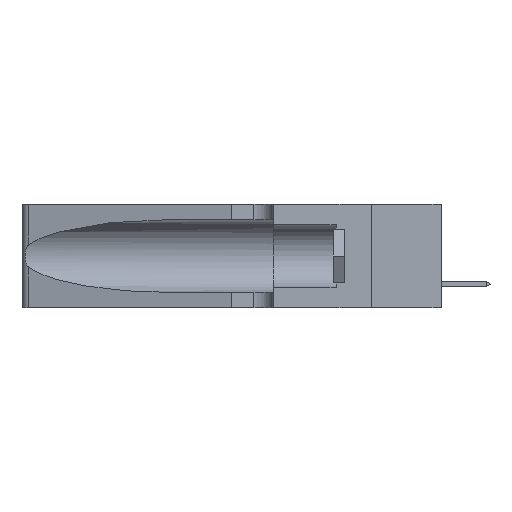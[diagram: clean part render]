
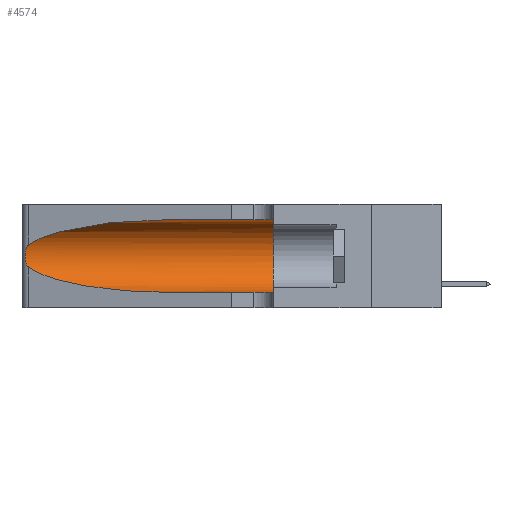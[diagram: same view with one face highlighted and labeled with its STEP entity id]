
A CAD part, left-side view. The second image highlights one B-rep face of the part: STEP entity #4574.
In plain terms, the highlighted cylindrical face has radius 3.308 mm (diameter 6.617 mm), a partial arc.
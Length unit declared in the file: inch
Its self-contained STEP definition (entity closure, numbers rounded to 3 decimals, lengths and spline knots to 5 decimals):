
#423 = CARTESIAN_POINT ( 'NONE',  ( 0.1305, 1.61858, 0.05475 ) ) ;
#582 = FACE_OUTER_BOUND ( 'NONE', #7957, .T. ) ;
#1213 = VERTEX_POINT ( 'NONE', #10068 ) ;
#1557 = EDGE_CURVE ( 'NONE', #7163, #1213, #6737, .T. ) ;
#1610 = CARTESIAN_POINT ( 'NONE',  ( 0.1305, 0.72297, 0.31525 ) ) ;
#2842 = CARTESIAN_POINT ( 'NONE',  ( 0.2373, 1.15595, 0.28018 ) ) ;
#3681 = ORIENTED_EDGE ( 'NONE', *, *, #4678, .T. ) ;
#3948 = CARTESIAN_POINT ( 'NONE',  ( 0.25787, 1.23484, 0.2124 ) ) ;
#4024 = CARTESIAN_POINT ( 'NONE',  ( 0.25555, 1.22993, 0.14849 ) ) ;
#4443 = ORIENTED_EDGE ( 'NONE', *, *, #22058, .F. ) ;
#4574 = ADVANCED_FACE ( 'NONE', ( #582 ), #6459, .F. ) ;
#4678 = EDGE_CURVE ( 'NONE', #1213, #16218, #20661, .T. ) ;
#4921 = CARTESIAN_POINT ( 'NONE',  ( 0.25487, 1.22718, 0.14631 ) ) ;
#6112 = CARTESIAN_POINT ( 'NONE',  ( 0.25487, 1.22718, 0.22369 ) ) ;
#6451 = VECTOR ( 'NONE', #15486, 39.37008 ) ;
#6459 = CYLINDRICAL_SURFACE ( 'NONE', #15802, 0.13025 ) ;
#6737 =( BOUNDED_CURVE ( )  B_SPLINE_CURVE ( 3, ( #4921, #11575, #7399, #14193 ),
 .UNSPECIFIED., .F., .T. ) 
 B_SPLINE_CURVE_WITH_KNOTS ( ( 4, 4 ),
 ( 3.44316, 4.71239 ),
 .UNSPECIFIED. ) 
 CURVE ( )  GEOMETRIC_REPRESENTATION_ITEM ( )  RATIONAL_B_SPLINE_CURVE ( ( 1., 0.87, 0.87, 1. ) ) 
 REPRESENTATION_ITEM ( '' )  );
#7163 = VERTEX_POINT ( 'NONE', #8894 ) ;
#7164 = CARTESIAN_POINT ( 'NONE',  ( 0.25487, 1.22718, 0.22369 ) ) ;
#7399 = CARTESIAN_POINT ( 'NONE',  ( 0.18966, 0.96281, 0.05475 ) ) ;
#7523 = DIRECTION ( 'NONE',  ( 0., 0., -1. ) ) ;
#7957 = EDGE_LOOP ( 'NONE', ( #8429, #14013, #21726, #3681, #17654, #4443 ) ) ;
#8325 = LINE ( 'NONE', #15269, #6451 ) ;
#8429 = ORIENTED_EDGE ( 'NONE', *, *, #15650, .T. ) ;
#8894 = CARTESIAN_POINT ( 'NONE',  ( 0.25487, 1.22718, 0.14631 ) ) ;
#9244 = VERTEX_POINT ( 'NONE', #6112 ) ;
#10068 = CARTESIAN_POINT ( 'NONE',  ( 0.1305, 0.72297, 0.05475 ) ) ;
#10772 = CARTESIAN_POINT ( 'NONE',  ( 0.25856, 1.23593, 0.16098 ) ) ;
#11281 = CARTESIAN_POINT ( 'NONE',  ( 0.25487, 1.22718, 0.22369 ) ) ;
#11575 = CARTESIAN_POINT ( 'NONE',  ( 0.2373, 1.15595, 0.08982 ) ) ;
#12140 = EDGE_CURVE ( 'NONE', #9244, #7163, #19660, .T. ) ;
#12554 = CARTESIAN_POINT ( 'NONE',  ( 0.26075, 1.23896, 0.178 ) ) ;
#12938 = AXIS2_PLACEMENT_3D ( 'NONE', #17990, #21541, #21406 ) ;
#13100 = CARTESIAN_POINT ( 'NONE',  ( 0.18966, 0.96281, 0.31525 ) ) ;
#13196 = VERTEX_POINT ( 'NONE', #1610 ) ;
#14013 = ORIENTED_EDGE ( 'NONE', *, *, #12140, .T. ) ;
#14113 = CARTESIAN_POINT ( 'NONE',  ( 0.25555, 1.22994, 0.2215 ) ) ;
#14164 = DIRECTION ( 'NONE',  ( 0., -1., 0. ) ) ;
#14193 = CARTESIAN_POINT ( 'NONE',  ( 0.1305, 0.72297, 0.05475 ) ) ;
#14201 = CARTESIAN_POINT ( 'NONE',  ( 0.25639, 1.23184, 0.21858 ) ) ;
#14276 = CARTESIAN_POINT ( 'NONE',  ( 0.25639, 1.23186, 0.15144 ) ) ;
#14664 = VERTEX_POINT ( 'NONE', #15324 ) ;
#14884 = CIRCLE ( 'NONE', #12938, 0.13025 ) ;
#15269 = CARTESIAN_POINT ( 'NONE',  ( 0.1305, 1.61858, 0.31525 ) ) ;
#15324 = CARTESIAN_POINT ( 'NONE',  ( 0.1305, 0.35, 0.31525 ) ) ;
#15486 = DIRECTION ( 'NONE',  ( 0., -1., 0. ) ) ;
#15650 = EDGE_CURVE ( 'NONE', #13196, #9244, #18834, .T. ) ;
#15802 = AXIS2_PLACEMENT_3D ( 'NONE', #19537, #14164, #7523 ) ;
#15947 = CARTESIAN_POINT ( 'NONE',  ( 0.25789, 1.23486, 0.15765 ) ) ;
#16003 = DIRECTION ( 'NONE',  ( 0., -1., 0. ) ) ;
#16024 = CARTESIAN_POINT ( 'NONE',  ( 0.25487, 1.22718, 0.14631 ) ) ;
#16122 = VECTOR ( 'NONE', #16003, 39.37008 ) ;
#16218 = VERTEX_POINT ( 'NONE', #20695 ) ;
#16785 = EDGE_CURVE ( 'NONE', #14664, #16218, #14884, .T. ) ;
#17654 = ORIENTED_EDGE ( 'NONE', *, *, #16785, .F. ) ;
#17990 = CARTESIAN_POINT ( 'NONE',  ( 0.1305, 0.35, 0.185 ) ) ;
#18834 =( BOUNDED_CURVE ( )  B_SPLINE_CURVE ( 3, ( #21545, #13100, #2842, #11281 ),
 .UNSPECIFIED., .F., .T. ) 
 B_SPLINE_CURVE_WITH_KNOTS ( ( 4, 4 ),
 ( 1.5708, 2.84003 ),
 .UNSPECIFIED. ) 
 CURVE ( )  GEOMETRIC_REPRESENTATION_ITEM ( )  RATIONAL_B_SPLINE_CURVE ( ( 1., 0.87, 0.87, 1. ) ) 
 REPRESENTATION_ITEM ( '' )  );
#19194 = CARTESIAN_POINT ( 'NONE',  ( 0.26075, 1.23896, 0.19203 ) ) ;
#19347 = CARTESIAN_POINT ( 'NONE',  ( 0.26018, 1.23835, 0.19895 ) ) ;
#19537 = CARTESIAN_POINT ( 'NONE',  ( 0.1305, 1.61858, 0.185 ) ) ;
#19660 = B_SPLINE_CURVE_WITH_KNOTS ( 'NONE', 3,
 ( #7164, #14113, #14201, #3948, #21093, #19347, #19194, #12554, #21014, #10772, #15947, #14276, #4024, #16024 ),
 .UNSPECIFIED., .F., .F.,
 ( 4, 2, 2, 2, 2, 2, 4 ),
 ( 0., 0.00027, 0.00053, 0.00107, 0.0016, 0.00187, 0.00214 ),
 .UNSPECIFIED. ) ;
#20661 = LINE ( 'NONE', #423, #16122 ) ;
#20695 = CARTESIAN_POINT ( 'NONE',  ( 0.1305, 0.35, 0.05475 ) ) ;
#21014 = CARTESIAN_POINT ( 'NONE',  ( 0.26017, 1.23833, 0.17102 ) ) ;
#21093 = CARTESIAN_POINT ( 'NONE',  ( 0.25854, 1.2359, 0.20912 ) ) ;
#21406 = DIRECTION ( 'NONE',  ( 0., 0., 1. ) ) ;
#21541 = DIRECTION ( 'NONE',  ( 0., 1., 0. ) ) ;
#21545 = CARTESIAN_POINT ( 'NONE',  ( 0.1305, 0.72297, 0.31525 ) ) ;
#21726 = ORIENTED_EDGE ( 'NONE', *, *, #1557, .T. ) ;
#22058 = EDGE_CURVE ( 'NONE', #13196, #14664, #8325, .T. ) ;
